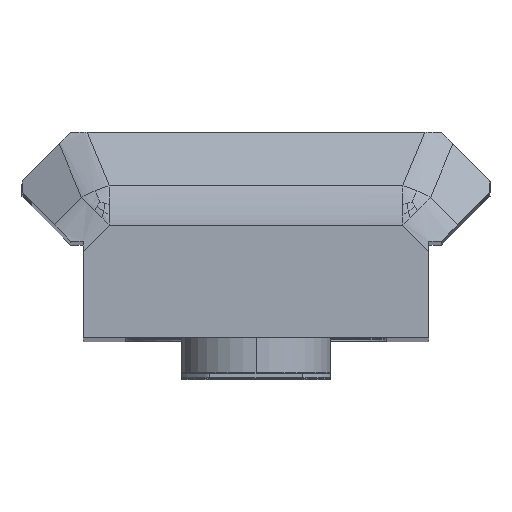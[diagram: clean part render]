
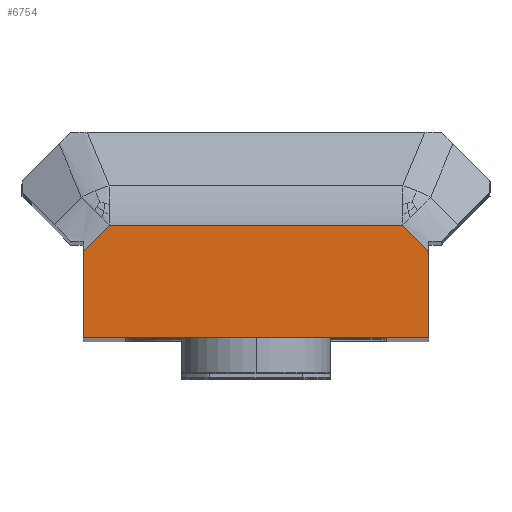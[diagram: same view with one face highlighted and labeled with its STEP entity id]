
A CAD part, top view. The second image highlights one B-rep face of the part: STEP entity #6754.
In plain terms, the highlighted planar face has unit normal (0, 0, 1).
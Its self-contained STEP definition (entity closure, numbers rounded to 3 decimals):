
#203 = CARTESIAN_POINT ( 'NONE',  ( -30.812, 18.14, 99.822 ) ) ;
#484 = CARTESIAN_POINT ( 'NONE',  ( -17.127, 18.538, 99.822 ) ) ;
#692 = ORIENTED_EDGE ( 'NONE', *, *, #7114, .T. ) ;
#1039 = CARTESIAN_POINT ( 'NONE',  ( -31.607, 13.443, 99.822 ) ) ;
#1060 = CARTESIAN_POINT ( 'NONE',  ( -30.415, 18.538, 99.822 ) ) ;
#1250 = DIRECTION ( 'NONE',  ( 0., 1., 0. ) ) ;
#1502 = CARTESIAN_POINT ( 'NONE',  ( -16.73, 18.14, 99.822 ) ) ;
#1851 = DIRECTION ( 'NONE',  ( 0., 0., 1. ) ) ;
#1940 = FACE_OUTER_BOUND ( 'NONE', #7290, .T. ) ;
#2014 = VERTEX_POINT ( 'NONE', #3948 ) ;
#2216 = CARTESIAN_POINT ( 'NONE',  ( -15.935, 17.346, 99.822 ) ) ;
#2260 = CARTESIAN_POINT ( 'NONE',  ( -16.333, 17.743, 99.822 ) ) ;
#2366 = B_SPLINE_CURVE_WITH_KNOTS ( 'NONE', 3,
 ( #2216, #2260, #1502, #6671 ),
 .UNSPECIFIED., .F., .F.,
 ( 4, 4 ),
 ( 0., 1. ),
 .UNSPECIFIED. ) ;
#2384 = VERTEX_POINT ( 'NONE', #2464 ) ;
#2464 = CARTESIAN_POINT ( 'NONE',  ( -15.935, 17.346, 99.822 ) ) ;
#2501 = CARTESIAN_POINT ( 'NONE',  ( -15.935, 13.443, 99.822 ) ) ;
#2530 = EDGE_CURVE ( 'NONE', #2384, #2014, #2366, .T. ) ;
#2559 = CARTESIAN_POINT ( 'NONE',  ( -31.607, 0., 99.822 ) ) ;
#2601 = VERTEX_POINT ( 'NONE', #8824 ) ;
#2793 = AXIS2_PLACEMENT_3D ( 'NONE', #7024, #1851, #5538 ) ;
#2794 = VERTEX_POINT ( 'NONE', #2501 ) ;
#3225 = VERTEX_POINT ( 'NONE', #3917 ) ;
#3279 = LINE ( 'NONE', #2559, #3781 ) ;
#3781 = VECTOR ( 'NONE', #7685, 1000. ) ;
#3825 = EDGE_CURVE ( 'NONE', #9462, #3225, #3279, .T. ) ;
#3917 = CARTESIAN_POINT ( 'NONE',  ( -31.607, 17.346, 99.822 ) ) ;
#3948 = CARTESIAN_POINT ( 'NONE',  ( -17.127, 18.538, 99.822 ) ) ;
#4073 = LINE ( 'NONE', #7004, #5016 ) ;
#4469 = ORIENTED_EDGE ( 'NONE', *, *, #7228, .T. ) ;
#4663 = B_SPLINE_CURVE_WITH_KNOTS ( 'NONE', 3,
 ( #1060, #203, #6862, #9064 ),
 .UNSPECIFIED., .F., .F.,
 ( 4, 4 ),
 ( 0., 1. ),
 .UNSPECIFIED. ) ;
#4768 = PLANE ( 'NONE',  #2793 ) ;
#4801 = ORIENTED_EDGE ( 'NONE', *, *, #8258, .T. ) ;
#4888 = CARTESIAN_POINT ( 'NONE',  ( -21.557, 18.538, 99.822 ) ) ;
#5016 = VECTOR ( 'NONE', #6378, 1000. ) ;
#5538 = DIRECTION ( 'NONE',  ( 1., 0., 0. ) ) ;
#5661 = LINE ( 'NONE', #9345, #6607 ) ;
#5808 = ORIENTED_EDGE ( 'NONE', *, *, #7978, .T. ) ;
#6062 = ORIENTED_EDGE ( 'NONE', *, *, #2530, .T. ) ;
#6378 = DIRECTION ( 'NONE',  ( 1., 0., 0. ) ) ;
#6470 = ORIENTED_EDGE ( 'NONE', *, *, #3825, .F. ) ;
#6607 = VECTOR ( 'NONE', #1250, 1000. ) ;
#6671 = CARTESIAN_POINT ( 'NONE',  ( -17.127, 18.538, 99.822 ) ) ;
#6754 = ADVANCED_FACE ( 'NONE', ( #1940 ), #4768, .T. ) ;
#6862 = CARTESIAN_POINT ( 'NONE',  ( -31.21, 17.743, 99.822 ) ) ;
#6896 = B_SPLINE_CURVE_WITH_KNOTS ( 'NONE', 3,
 ( #484, #4888, #9197, #7095 ),
 .UNSPECIFIED., .F., .F.,
 ( 4, 4 ),
 ( 0., 1. ),
 .UNSPECIFIED. ) ;
#7004 = CARTESIAN_POINT ( 'NONE',  ( 0., 13.443, 99.822 ) ) ;
#7024 = CARTESIAN_POINT ( 'NONE',  ( 0., 0., 99.822 ) ) ;
#7095 = CARTESIAN_POINT ( 'NONE',  ( -30.415, 18.538, 99.822 ) ) ;
#7114 = EDGE_CURVE ( 'NONE', #2794, #2384, #5661, .T. ) ;
#7228 = EDGE_CURVE ( 'NONE', #2014, #2601, #6896, .T. ) ;
#7290 = EDGE_LOOP ( 'NONE', ( #4469, #5808, #6470, #4801, #692, #6062 ) ) ;
#7685 = DIRECTION ( 'NONE',  ( 0., 1., 0. ) ) ;
#7978 = EDGE_CURVE ( 'NONE', #2601, #3225, #4663, .T. ) ;
#8258 = EDGE_CURVE ( 'NONE', #9462, #2794, #4073, .T. ) ;
#8824 = CARTESIAN_POINT ( 'NONE',  ( -30.415, 18.538, 99.822 ) ) ;
#9064 = CARTESIAN_POINT ( 'NONE',  ( -31.607, 17.346, 99.822 ) ) ;
#9197 = CARTESIAN_POINT ( 'NONE',  ( -25.986, 18.538, 99.822 ) ) ;
#9345 = CARTESIAN_POINT ( 'NONE',  ( -15.935, 0., 99.822 ) ) ;
#9462 = VERTEX_POINT ( 'NONE', #1039 ) ;
